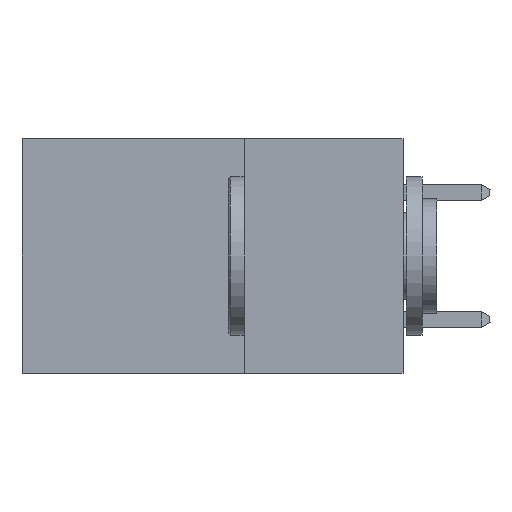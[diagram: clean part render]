
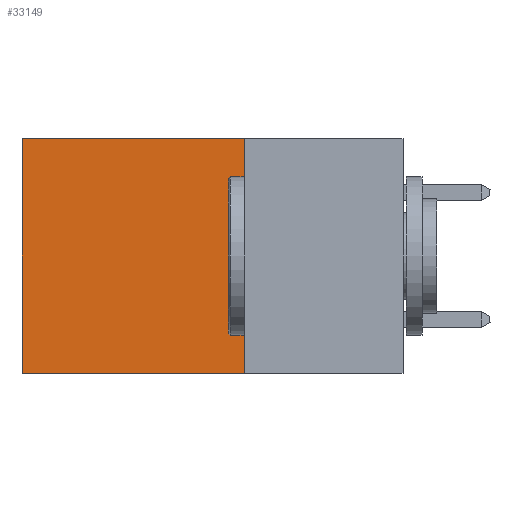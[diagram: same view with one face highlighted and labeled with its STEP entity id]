
A CAD part, left-side view. The second image highlights one B-rep face of the part: STEP entity #33149.
In plain terms, the highlighted planar face has unit normal (-1, 0, 0).
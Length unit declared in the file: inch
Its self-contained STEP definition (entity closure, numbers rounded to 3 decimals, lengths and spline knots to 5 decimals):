
#1301 = CARTESIAN_POINT ( 'NONE',  ( 0.2875, 0.25, 0. ) ) ;
#3213 = VERTEX_POINT ( 'NONE', #34781 ) ;
#4786 = EDGE_CURVE ( 'NONE', #3213, #32675, #9526, .T. ) ;
#4988 = ORIENTED_EDGE ( 'NONE', *, *, #27721, .T. ) ;
#5519 = DIRECTION ( 'NONE',  ( 0., 1., 0. ) ) ;
#5711 = VECTOR ( 'NONE', #5519, 39.37008 ) ;
#9526 = LINE ( 'NONE', #38743, #25797 ) ;
#11280 = VECTOR ( 'NONE', #22068, 39.37008 ) ;
#12514 = LINE ( 'NONE', #15121, #27790 ) ;
#14877 = EDGE_CURVE ( 'NONE', #38337, #3213, #12514, .T. ) ;
#15121 = CARTESIAN_POINT ( 'NONE',  ( 0.2875, 0.25, 0. ) ) ;
#15254 = ORIENTED_EDGE ( 'NONE', *, *, #20681, .T. ) ;
#16499 = DIRECTION ( 'NONE',  ( 1., 0., 0. ) ) ;
#18223 = DIRECTION ( 'NONE',  ( 0., 0., -1. ) ) ;
#18479 = LINE ( 'NONE', #19008, #11280 ) ;
#19008 = CARTESIAN_POINT ( 'NONE',  ( 0.2875, 0.6, 0. ) ) ;
#20179 = VERTEX_POINT ( 'NONE', #27342 ) ;
#20646 = DIRECTION ( 'NONE',  ( 0., 1., 0. ) ) ;
#20681 = EDGE_CURVE ( 'NONE', #38337, #20179, #38056, .T. ) ;
#22068 = DIRECTION ( 'NONE',  ( 0., 0., -1. ) ) ;
#22943 = FACE_OUTER_BOUND ( 'NONE', #26725, .T. ) ;
#23467 = CARTESIAN_POINT ( 'NONE',  ( 0.2875, 0.6, -0.37 ) ) ;
#25565 = PLANE ( 'NONE',  #27337 ) ;
#25598 = ORIENTED_EDGE ( 'NONE', *, *, #4786, .F. ) ;
#25797 = VECTOR ( 'NONE', #20646, 39.37008 ) ;
#26725 = EDGE_LOOP ( 'NONE', ( #4988, #25598, #31378, #15254 ) ) ;
#27337 = AXIS2_PLACEMENT_3D ( 'NONE', #34662, #16499, #37684 ) ;
#27342 = CARTESIAN_POINT ( 'NONE',  ( 0.2875, 0.6, 0. ) ) ;
#27721 = EDGE_CURVE ( 'NONE', #20179, #32675, #18479, .T. ) ;
#27790 = VECTOR ( 'NONE', #18223, 39.37008 ) ;
#31378 = ORIENTED_EDGE ( 'NONE', *, *, #14877, .F. ) ;
#32675 = VERTEX_POINT ( 'NONE', #23467 ) ;
#33149 = ADVANCED_FACE ( 'NONE', ( #22943 ), #25565, .F. ) ;
#34662 = CARTESIAN_POINT ( 'NONE',  ( 0.2875, 0.25, 0. ) ) ;
#34781 = CARTESIAN_POINT ( 'NONE',  ( 0.2875, 0.25, -0.37 ) ) ;
#35880 = CARTESIAN_POINT ( 'NONE',  ( 0.2875, 0.25, 0. ) ) ;
#37684 = DIRECTION ( 'NONE',  ( 0., 0., -1. ) ) ;
#38056 = LINE ( 'NONE', #35880, #5711 ) ;
#38337 = VERTEX_POINT ( 'NONE', #1301 ) ;
#38743 = CARTESIAN_POINT ( 'NONE',  ( 0.2875, 0.25, -0.37 ) ) ;
